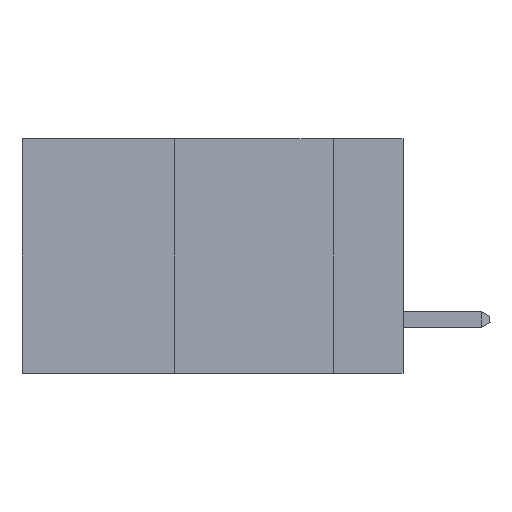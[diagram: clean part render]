
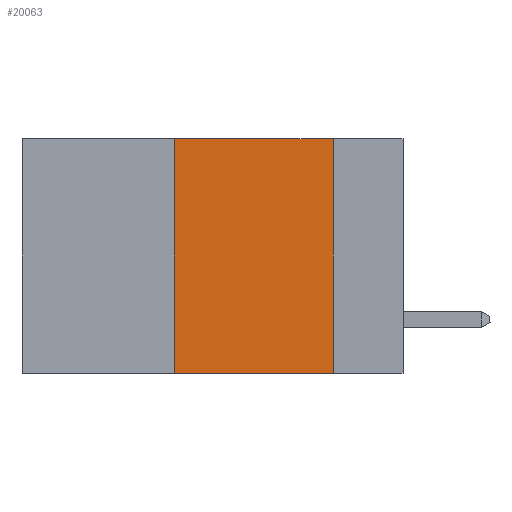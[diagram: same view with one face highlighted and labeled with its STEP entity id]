
A CAD part, left-side view. The second image highlights one B-rep face of the part: STEP entity #20063.
In plain terms, the highlighted planar face has unit normal (-1, 0, 0).
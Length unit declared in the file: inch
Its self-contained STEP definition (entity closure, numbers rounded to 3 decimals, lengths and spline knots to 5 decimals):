
#405 = CARTESIAN_POINT ( 'NONE',  ( 0., 0.36, -0.37 ) ) ;
#641 = CARTESIAN_POINT ( 'NONE',  ( 0., 0.6, 0. ) ) ;
#1169 = LINE ( 'NONE', #10273, #17292 ) ;
#2341 = VERTEX_POINT ( 'NONE', #17689 ) ;
#2647 = VECTOR ( 'NONE', #16931, 39.37008 ) ;
#3348 = ORIENTED_EDGE ( 'NONE', *, *, #19622, .F. ) ;
#3965 = EDGE_CURVE ( 'NONE', #8972, #21378, #20267, .T. ) ;
#4502 = CARTESIAN_POINT ( 'NONE',  ( 0., 0.36, 0. ) ) ;
#5336 = ORIENTED_EDGE ( 'NONE', *, *, #3965, .F. ) ;
#5469 = EDGE_CURVE ( 'NONE', #20849, #21378, #1169, .T. ) ;
#6498 = DIRECTION ( 'NONE',  ( 0., 0., 1. ) ) ;
#6808 = CARTESIAN_POINT ( 'NONE',  ( 0., 0.6, 0. ) ) ;
#7216 = ORIENTED_EDGE ( 'NONE', *, *, #5469, .T. ) ;
#7808 = VECTOR ( 'NONE', #6498, 39.37008 ) ;
#8160 = CARTESIAN_POINT ( 'NONE',  ( 0., 0.11, 0. ) ) ;
#8972 = VERTEX_POINT ( 'NONE', #8160 ) ;
#9118 = CARTESIAN_POINT ( 'NONE',  ( 0., 0.11, 0. ) ) ;
#10273 = CARTESIAN_POINT ( 'NONE',  ( 0., 0.6, -0.37 ) ) ;
#10679 = DIRECTION ( 'NONE',  ( 0., 0., -1. ) ) ;
#11060 = EDGE_CURVE ( 'NONE', #2341, #8972, #12163, .T. ) ;
#12163 = LINE ( 'NONE', #6808, #2647 ) ;
#12496 = DIRECTION ( 'NONE',  ( 1., 0., 0. ) ) ;
#13043 = LINE ( 'NONE', #4502, #7808 ) ;
#13046 = EDGE_LOOP ( 'NONE', ( #5336, #15444, #3348, #7216 ) ) ;
#14195 = DIRECTION ( 'NONE',  ( 0., 0., -1. ) ) ;
#15444 = ORIENTED_EDGE ( 'NONE', *, *, #11060, .F. ) ;
#15836 = VECTOR ( 'NONE', #10679, 39.37008 ) ;
#16931 = DIRECTION ( 'NONE',  ( 0., -1., 0. ) ) ;
#17292 = VECTOR ( 'NONE', #18844, 39.37008 ) ;
#17689 = CARTESIAN_POINT ( 'NONE',  ( 0., 0.36, 0. ) ) ;
#18765 = CARTESIAN_POINT ( 'NONE',  ( 0., 0.11, -0.37 ) ) ;
#18844 = DIRECTION ( 'NONE',  ( 0., -1., 0. ) ) ;
#19622 = EDGE_CURVE ( 'NONE', #20849, #2341, #13043, .T. ) ;
#20063 = ADVANCED_FACE ( 'NONE', ( #20382 ), #21006, .F. ) ;
#20267 = LINE ( 'NONE', #9118, #15836 ) ;
#20382 = FACE_OUTER_BOUND ( 'NONE', #13046, .T. ) ;
#20849 = VERTEX_POINT ( 'NONE', #405 ) ;
#21006 = PLANE ( 'NONE',  #21078 ) ;
#21078 = AXIS2_PLACEMENT_3D ( 'NONE', #641, #12496, #14195 ) ;
#21378 = VERTEX_POINT ( 'NONE', #18765 ) ;
